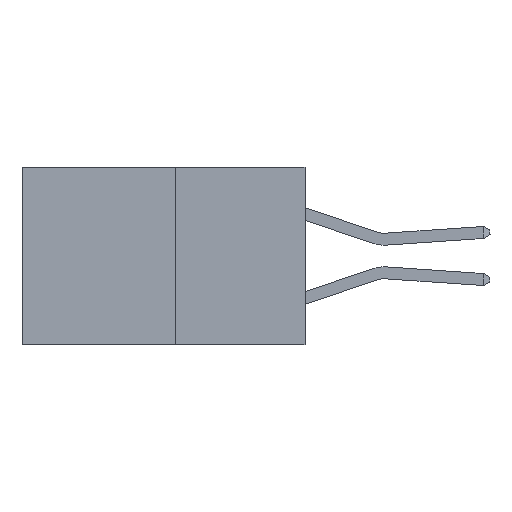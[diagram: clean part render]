
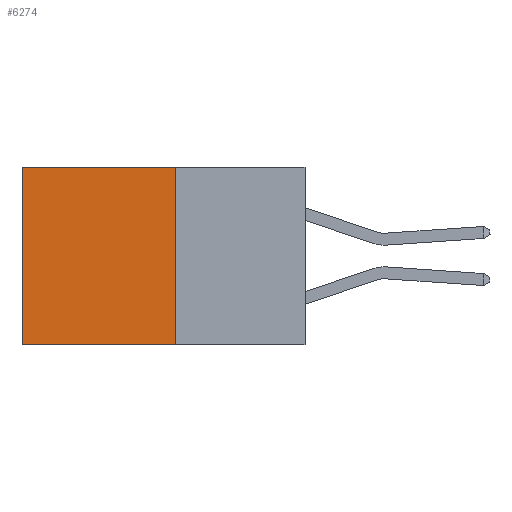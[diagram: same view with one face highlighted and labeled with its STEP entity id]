
A CAD part, left-side view. The second image highlights one B-rep face of the part: STEP entity #6274.
In plain terms, the highlighted planar face has unit normal (-1, 0, 0).
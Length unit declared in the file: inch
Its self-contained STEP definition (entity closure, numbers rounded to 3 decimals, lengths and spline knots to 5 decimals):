
#191 = CARTESIAN_POINT ( 'NONE',  ( 0.277, 0.27, -0.37 ) ) ;
#233 = DIRECTION ( 'NONE',  ( 0., 1., 0. ) ) ;
#453 = ORIENTED_EDGE ( 'NONE', *, *, #9592, .T. ) ;
#494 = DIRECTION ( 'NONE',  ( 0., 0., -1. ) ) ;
#539 = DIRECTION ( 'NONE',  ( 1., 0., 0. ) ) ;
#577 = PLANE ( 'NONE',  #1799 ) ;
#593 = CARTESIAN_POINT ( 'NONE',  ( 0.277, 0.59, -0.37 ) ) ;
#621 = CARTESIAN_POINT ( 'NONE',  ( 0.277, 0.27, -0.37 ) ) ;
#946 = ORIENTED_EDGE ( 'NONE', *, *, #7716, .F. ) ;
#1215 = EDGE_CURVE ( 'NONE', #1557, #2492, #10356, .T. ) ;
#1536 = LINE ( 'NONE', #593, #3901 ) ;
#1557 = VERTEX_POINT ( 'NONE', #3451 ) ;
#1799 = AXIS2_PLACEMENT_3D ( 'NONE', #621, #539, #494 ) ;
#2120 = EDGE_CURVE ( 'NONE', #10512, #4581, #1536, .T. ) ;
#2408 = ORIENTED_EDGE ( 'NONE', *, *, #1215, .F. ) ;
#2464 = ORIENTED_EDGE ( 'NONE', *, *, #2120, .T. ) ;
#2492 = VERTEX_POINT ( 'NONE', #6568 ) ;
#2893 = CARTESIAN_POINT ( 'NONE',  ( 0.277, 0.27, 0. ) ) ;
#3451 = CARTESIAN_POINT ( 'NONE',  ( 0.277, 0.27, 0. ) ) ;
#3458 = VECTOR ( 'NONE', #9009, 39.37008 ) ;
#3506 = VECTOR ( 'NONE', #7162, 39.37008 ) ;
#3901 = VECTOR ( 'NONE', #10904, 39.37008 ) ;
#4581 = VERTEX_POINT ( 'NONE', #9569 ) ;
#4715 = LINE ( 'NONE', #191, #9083 ) ;
#4747 = EDGE_LOOP ( 'NONE', ( #2464, #946, #2408, #453 ) ) ;
#6274 = ADVANCED_FACE ( 'NONE', ( #10668 ), #577, .F. ) ;
#6568 = CARTESIAN_POINT ( 'NONE',  ( 0.277, 0.27, -0.37 ) ) ;
#7162 = DIRECTION ( 'NONE',  ( 0., 0., -1. ) ) ;
#7716 = EDGE_CURVE ( 'NONE', #2492, #4581, #4715, .T. ) ;
#8542 = CARTESIAN_POINT ( 'NONE',  ( 0.277, 0.27, -0.37 ) ) ;
#9009 = DIRECTION ( 'NONE',  ( 0., 1., 0. ) ) ;
#9083 = VECTOR ( 'NONE', #233, 39.37008 ) ;
#9569 = CARTESIAN_POINT ( 'NONE',  ( 0.277, 0.59, -0.37 ) ) ;
#9576 = CARTESIAN_POINT ( 'NONE',  ( 0.277, 0.59, 0. ) ) ;
#9592 = EDGE_CURVE ( 'NONE', #1557, #10512, #9827, .T. ) ;
#9827 = LINE ( 'NONE', #2893, #3458 ) ;
#10356 = LINE ( 'NONE', #8542, #3506 ) ;
#10512 = VERTEX_POINT ( 'NONE', #9576 ) ;
#10668 = FACE_OUTER_BOUND ( 'NONE', #4747, .T. ) ;
#10904 = DIRECTION ( 'NONE',  ( 0., 0., -1. ) ) ;
